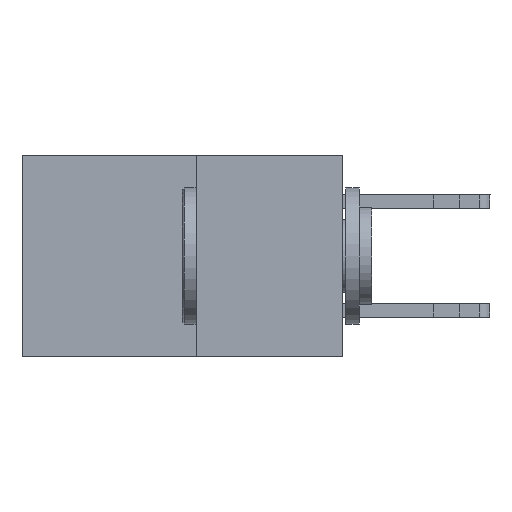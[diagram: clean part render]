
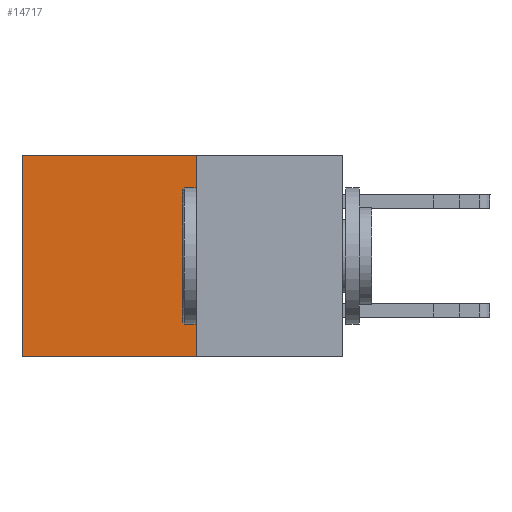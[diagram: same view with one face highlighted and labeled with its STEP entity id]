
A CAD part, left-side view. The second image highlights one B-rep face of the part: STEP entity #14717.
In plain terms, the highlighted planar face has unit normal (-1, 0, 0).
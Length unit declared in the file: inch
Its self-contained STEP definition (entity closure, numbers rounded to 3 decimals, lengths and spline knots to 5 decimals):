
#1901 = AXIS2_PLACEMENT_3D ( 'NONE', #14048, #15794, #7837 ) ;
#2787 = CARTESIAN_POINT ( 'NONE',  ( 0.277, 0.59, 0. ) ) ;
#3650 = CARTESIAN_POINT ( 'NONE',  ( 0.277, 0.59, -0.37 ) ) ;
#4105 = LINE ( 'NONE', #3650, #24819 ) ;
#5425 = VECTOR ( 'NONE', #16897, 39.37008 ) ;
#6041 = EDGE_CURVE ( 'NONE', #7313, #20900, #4105, .T. ) ;
#6266 = VERTEX_POINT ( 'NONE', #20012 ) ;
#6459 = FACE_OUTER_BOUND ( 'NONE', #22498, .T. ) ;
#7298 = EDGE_CURVE ( 'NONE', #6266, #7313, #22109, .T. ) ;
#7313 = VERTEX_POINT ( 'NONE', #2787 ) ;
#7562 = ORIENTED_EDGE ( 'NONE', *, *, #10540, .F. ) ;
#7672 = VECTOR ( 'NONE', #21848, 39.37008 ) ;
#7837 = DIRECTION ( 'NONE',  ( 0., 0., -1. ) ) ;
#9376 = DIRECTION ( 'NONE',  ( 0., 0., -1. ) ) ;
#9558 = CARTESIAN_POINT ( 'NONE',  ( 0.277, 0.27, -0.37 ) ) ;
#9904 = DIRECTION ( 'NONE',  ( 0., 0., -1. ) ) ;
#10080 = VERTEX_POINT ( 'NONE', #17976 ) ;
#10540 = EDGE_CURVE ( 'NONE', #6266, #10080, #17224, .T. ) ;
#11149 = ORIENTED_EDGE ( 'NONE', *, *, #6041, .T. ) ;
#11446 = LINE ( 'NONE', #9558, #5425 ) ;
#11658 = CARTESIAN_POINT ( 'NONE',  ( 0.277, 0.59, -0.37 ) ) ;
#13085 = VECTOR ( 'NONE', #9376, 39.37008 ) ;
#14048 = CARTESIAN_POINT ( 'NONE',  ( 0.277, 0.27, -0.37 ) ) ;
#14319 = ORIENTED_EDGE ( 'NONE', *, *, #17239, .F. ) ;
#14717 = ADVANCED_FACE ( 'NONE', ( #6459 ), #23275, .F. ) ;
#15775 = CARTESIAN_POINT ( 'NONE',  ( 0.277, 0.27, 0. ) ) ;
#15794 = DIRECTION ( 'NONE',  ( 1., 0., 0. ) ) ;
#16897 = DIRECTION ( 'NONE',  ( 0., 1., 0. ) ) ;
#17224 = LINE ( 'NONE', #18734, #13085 ) ;
#17239 = EDGE_CURVE ( 'NONE', #10080, #20900, #11446, .T. ) ;
#17779 = ORIENTED_EDGE ( 'NONE', *, *, #7298, .T. ) ;
#17976 = CARTESIAN_POINT ( 'NONE',  ( 0.277, 0.27, -0.37 ) ) ;
#18734 = CARTESIAN_POINT ( 'NONE',  ( 0.277, 0.27, -0.37 ) ) ;
#20012 = CARTESIAN_POINT ( 'NONE',  ( 0.277, 0.27, 0. ) ) ;
#20900 = VERTEX_POINT ( 'NONE', #11658 ) ;
#21848 = DIRECTION ( 'NONE',  ( 0., 1., 0. ) ) ;
#22109 = LINE ( 'NONE', #15775, #7672 ) ;
#22498 = EDGE_LOOP ( 'NONE', ( #11149, #14319, #7562, #17779 ) ) ;
#23275 = PLANE ( 'NONE',  #1901 ) ;
#24819 = VECTOR ( 'NONE', #9904, 39.37008 ) ;
